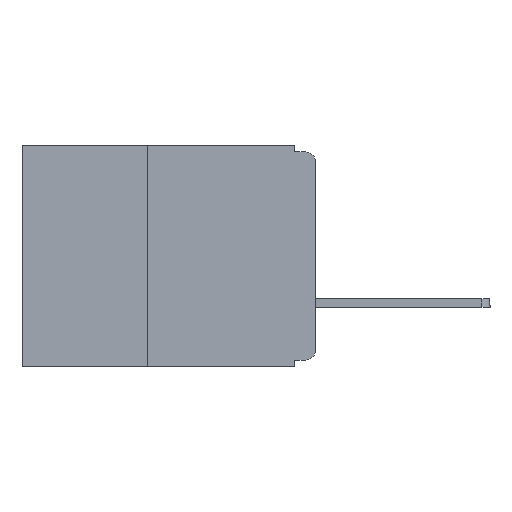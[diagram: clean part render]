
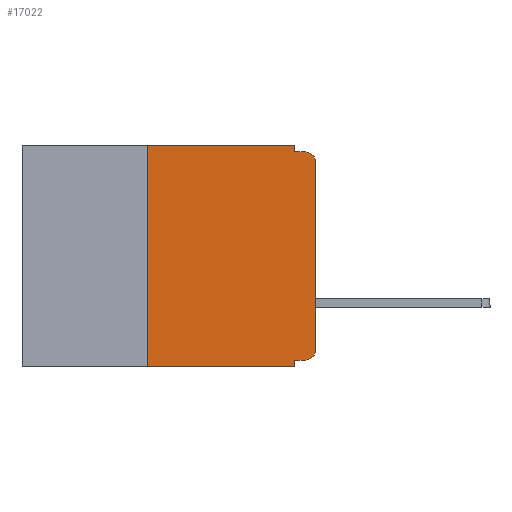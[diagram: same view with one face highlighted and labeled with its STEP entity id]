
A CAD part, left-side view. The second image highlights one B-rep face of the part: STEP entity #17022.
In plain terms, the highlighted planar face has unit normal (-1, 0, 0).
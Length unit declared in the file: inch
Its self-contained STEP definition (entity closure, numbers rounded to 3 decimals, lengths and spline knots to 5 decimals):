
#215 = VECTOR ( 'NONE', #17049, 39.37008 ) ;
#425 = CARTESIAN_POINT ( 'NONE',  ( 0., 0.437, 0. ) ) ;
#1077 = VERTEX_POINT ( 'NONE', #4390 ) ;
#1171 = CARTESIAN_POINT ( 'NONE',  ( 0., 0.25, -0.33 ) ) ;
#1208 = EDGE_CURVE ( 'NONE', #13954, #19519, #8207, .T. ) ;
#1307 = LINE ( 'NONE', #1171, #215 ) ;
#1340 = CARTESIAN_POINT ( 'NONE',  ( 0., 0.437, 0. ) ) ;
#1998 = EDGE_LOOP ( 'NONE', ( #12781, #17975, #8614, #20694, #16653, #14216, #19398, #12291, #3999, #5070 ) ) ;
#2479 = CARTESIAN_POINT ( 'NONE',  ( 0., 0.015, -0.32 ) ) ;
#2605 = DIRECTION ( 'NONE',  ( 0., 0., 1. ) ) ;
#2742 = LINE ( 'NONE', #13725, #11601 ) ;
#3026 = VERTEX_POINT ( 'NONE', #22270 ) ;
#3279 = CARTESIAN_POINT ( 'NONE',  ( 0., 0., 0. ) ) ;
#3295 = DIRECTION ( 'NONE',  ( -1., 0., 0. ) ) ;
#3780 = VERTEX_POINT ( 'NONE', #2479 ) ;
#3999 = ORIENTED_EDGE ( 'NONE', *, *, #21167, .F. ) ;
#4294 = EDGE_CURVE ( 'NONE', #7671, #9297, #13868, .T. ) ;
#4390 = CARTESIAN_POINT ( 'NONE',  ( 0., 0.25, -0.33 ) ) ;
#4734 = VERTEX_POINT ( 'NONE', #8723 ) ;
#4944 = CIRCLE ( 'NONE', #5547, 0.015 ) ;
#4983 = EDGE_CURVE ( 'NONE', #9297, #7165, #21163, .T. ) ;
#5070 = ORIENTED_EDGE ( 'NONE', *, *, #22449, .T. ) ;
#5547 = AXIS2_PLACEMENT_3D ( 'NONE', #13898, #3295, #15658 ) ;
#5780 = VECTOR ( 'NONE', #12749, 39.37008 ) ;
#5992 = CARTESIAN_POINT ( 'NONE',  ( 0., 0.031, 0. ) ) ;
#6295 = EDGE_CURVE ( 'NONE', #1077, #7671, #1307, .T. ) ;
#6633 = PLANE ( 'NONE',  #9317 ) ;
#6793 = LINE ( 'NONE', #21650, #7913 ) ;
#7165 = VERTEX_POINT ( 'NONE', #19736 ) ;
#7528 = VERTEX_POINT ( 'NONE', #22423 ) ;
#7671 = VERTEX_POINT ( 'NONE', #21068 ) ;
#7913 = VECTOR ( 'NONE', #19934, 39.37008 ) ;
#8207 = LINE ( 'NONE', #3279, #17035 ) ;
#8431 = DIRECTION ( 'NONE',  ( -1., 0., 0. ) ) ;
#8432 = DIRECTION ( 'NONE',  ( 0., 0., -1. ) ) ;
#8614 = ORIENTED_EDGE ( 'NONE', *, *, #18871, .F. ) ;
#8723 = CARTESIAN_POINT ( 'NONE',  ( 0., 0.015, -0.01 ) ) ;
#9090 = CARTESIAN_POINT ( 'NONE',  ( 0., 0.031, -0.33 ) ) ;
#9297 = VERTEX_POINT ( 'NONE', #10158 ) ;
#9317 = AXIS2_PLACEMENT_3D ( 'NONE', #1340, #18983, #8432 ) ;
#9549 = CARTESIAN_POINT ( 'NONE',  ( 0., 0., -0.025 ) ) ;
#9862 = DIRECTION ( 'NONE',  ( 0., 1., 0. ) ) ;
#10158 = CARTESIAN_POINT ( 'NONE',  ( 0., 0.031, 0. ) ) ;
#10512 = LINE ( 'NONE', #9090, #5780 ) ;
#10900 = EDGE_CURVE ( 'NONE', #7528, #3026, #10512, .T. ) ;
#11019 = DIRECTION ( 'NONE',  ( 0., -1., 0. ) ) ;
#11246 = EDGE_CURVE ( 'NONE', #1077, #3026, #2742, .T. ) ;
#11601 = VECTOR ( 'NONE', #15494, 39.37008 ) ;
#11743 = EDGE_CURVE ( 'NONE', #19519, #4734, #19787, .T. ) ;
#11802 = CARTESIAN_POINT ( 'NONE',  ( 0., 0., -0.32 ) ) ;
#12291 = ORIENTED_EDGE ( 'NONE', *, *, #10900, .F. ) ;
#12749 = DIRECTION ( 'NONE',  ( 0., 0., -1. ) ) ;
#12781 = ORIENTED_EDGE ( 'NONE', *, *, #1208, .T. ) ;
#13725 = CARTESIAN_POINT ( 'NONE',  ( 0., 0.437, -0.33 ) ) ;
#13868 = LINE ( 'NONE', #425, #22545 ) ;
#13898 = CARTESIAN_POINT ( 'NONE',  ( 0., 0.015, -0.305 ) ) ;
#13954 = VERTEX_POINT ( 'NONE', #21365 ) ;
#14216 = ORIENTED_EDGE ( 'NONE', *, *, #6295, .F. ) ;
#14832 = DIRECTION ( 'NONE',  ( 0., 0., -1. ) ) ;
#15494 = DIRECTION ( 'NONE',  ( 0., -1., 0. ) ) ;
#15658 = DIRECTION ( 'NONE',  ( 0., 0., -1. ) ) ;
#16653 = ORIENTED_EDGE ( 'NONE', *, *, #4294, .F. ) ;
#17022 = ADVANCED_FACE ( 'NONE', ( #22529 ), #6633, .F. ) ;
#17035 = VECTOR ( 'NONE', #2605, 39.37008 ) ;
#17049 = DIRECTION ( 'NONE',  ( 0., 0., 1. ) ) ;
#17462 = LINE ( 'NONE', #11802, #20966 ) ;
#17654 = AXIS2_PLACEMENT_3D ( 'NONE', #18981, #8431, #20691 ) ;
#17975 = ORIENTED_EDGE ( 'NONE', *, *, #11743, .T. ) ;
#18871 = EDGE_CURVE ( 'NONE', #7165, #4734, #6793, .T. ) ;
#18981 = CARTESIAN_POINT ( 'NONE',  ( 0., 0.015, -0.025 ) ) ;
#18983 = DIRECTION ( 'NONE',  ( 1., 0., 0. ) ) ;
#19398 = ORIENTED_EDGE ( 'NONE', *, *, #11246, .T. ) ;
#19519 = VERTEX_POINT ( 'NONE', #9549 ) ;
#19736 = CARTESIAN_POINT ( 'NONE',  ( 0., 0.031, -0.01 ) ) ;
#19787 = CIRCLE ( 'NONE', #17654, 0.015 ) ;
#19934 = DIRECTION ( 'NONE',  ( 0., -1., 0. ) ) ;
#20612 = VECTOR ( 'NONE', #14832, 39.37008 ) ;
#20691 = DIRECTION ( 'NONE',  ( 0., 0., -1. ) ) ;
#20694 = ORIENTED_EDGE ( 'NONE', *, *, #4983, .F. ) ;
#20966 = VECTOR ( 'NONE', #9862, 39.37008 ) ;
#21068 = CARTESIAN_POINT ( 'NONE',  ( 0., 0.25, 0. ) ) ;
#21163 = LINE ( 'NONE', #5992, #20612 ) ;
#21167 = EDGE_CURVE ( 'NONE', #3780, #7528, #17462, .T. ) ;
#21365 = CARTESIAN_POINT ( 'NONE',  ( 0., 0., -0.305 ) ) ;
#21650 = CARTESIAN_POINT ( 'NONE',  ( 0., 0., -0.01 ) ) ;
#22270 = CARTESIAN_POINT ( 'NONE',  ( 0., 0.031, -0.33 ) ) ;
#22423 = CARTESIAN_POINT ( 'NONE',  ( 0., 0.031, -0.32 ) ) ;
#22449 = EDGE_CURVE ( 'NONE', #3780, #13954, #4944, .T. ) ;
#22529 = FACE_OUTER_BOUND ( 'NONE', #1998, .T. ) ;
#22545 = VECTOR ( 'NONE', #11019, 39.37008 ) ;
